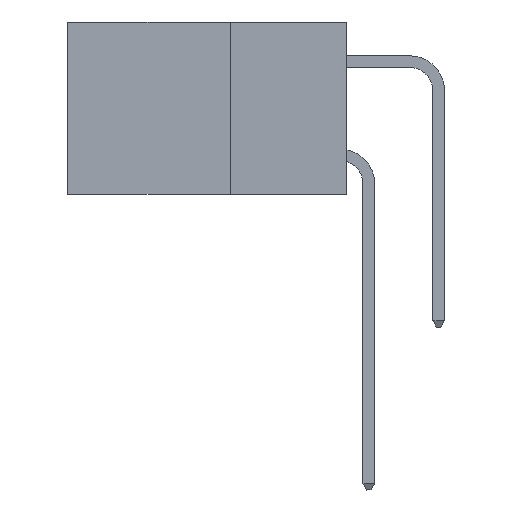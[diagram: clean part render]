
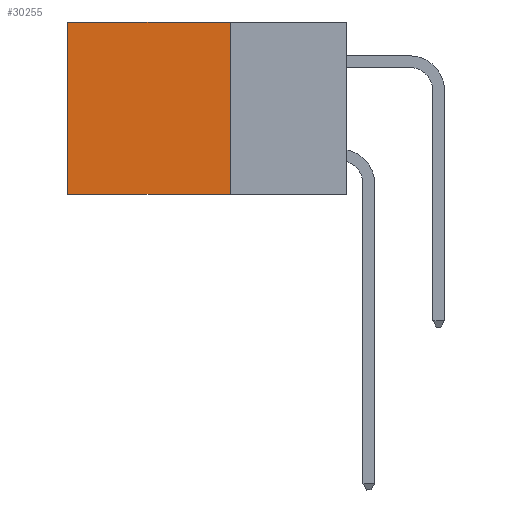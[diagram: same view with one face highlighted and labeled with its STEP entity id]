
A CAD part, left-side view. The second image highlights one B-rep face of the part: STEP entity #30255.
In plain terms, the highlighted planar face has unit normal (-1, 0, 0).
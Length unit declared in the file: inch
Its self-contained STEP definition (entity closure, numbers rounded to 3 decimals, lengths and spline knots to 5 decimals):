
#348 = VERTEX_POINT ( 'NONE', #10802 ) ;
#1206 = CARTESIAN_POINT ( 'NONE',  ( 0.2875, 0.25, 0. ) ) ;
#1921 = VECTOR ( 'NONE', #30288, 39.37008 ) ;
#4681 = EDGE_CURVE ( 'NONE', #19000, #29378, #31985, .T. ) ;
#5032 = DIRECTION ( 'NONE',  ( 1., 0., 0. ) ) ;
#6485 = EDGE_CURVE ( 'NONE', #29378, #12026, #27161, .T. ) ;
#6731 = VECTOR ( 'NONE', #34217, 39.37008 ) ;
#9121 = LINE ( 'NONE', #19174, #1921 ) ;
#9822 = ORIENTED_EDGE ( 'NONE', *, *, #4681, .F. ) ;
#9982 = CARTESIAN_POINT ( 'NONE',  ( 0.2875, 0.25, -0.37 ) ) ;
#10748 = FACE_OUTER_BOUND ( 'NONE', #27611, .T. ) ;
#10802 = CARTESIAN_POINT ( 'NONE',  ( 0.2875, 0.6, 0. ) ) ;
#10905 = EDGE_CURVE ( 'NONE', #348, #12026, #35286, .T. ) ;
#12026 = VERTEX_POINT ( 'NONE', #22882 ) ;
#12740 = EDGE_CURVE ( 'NONE', #19000, #348, #9121, .T. ) ;
#13282 = VECTOR ( 'NONE', #24494, 39.37008 ) ;
#14138 = ORIENTED_EDGE ( 'NONE', *, *, #10905, .T. ) ;
#14485 = DIRECTION ( 'NONE',  ( 0., 0., -1. ) ) ;
#15647 = VECTOR ( 'NONE', #14485, 39.37008 ) ;
#17063 = CARTESIAN_POINT ( 'NONE',  ( 0.2875, 0.25, -0.37 ) ) ;
#17558 = CARTESIAN_POINT ( 'NONE',  ( 0.2875, 0.25, 0. ) ) ;
#19000 = VERTEX_POINT ( 'NONE', #1206 ) ;
#19174 = CARTESIAN_POINT ( 'NONE',  ( 0.2875, 0.25, 0. ) ) ;
#20976 = DIRECTION ( 'NONE',  ( 0., 0., -1. ) ) ;
#22882 = CARTESIAN_POINT ( 'NONE',  ( 0.2875, 0.6, -0.37 ) ) ;
#23596 = PLANE ( 'NONE',  #23785 ) ;
#23785 = AXIS2_PLACEMENT_3D ( 'NONE', #34789, #5032, #20976 ) ;
#24494 = DIRECTION ( 'NONE',  ( 0., 0., -1. ) ) ;
#25568 = ORIENTED_EDGE ( 'NONE', *, *, #6485, .F. ) ;
#27161 = LINE ( 'NONE', #9982, #6731 ) ;
#27611 = EDGE_LOOP ( 'NONE', ( #14138, #25568, #9822, #29611 ) ) ;
#27710 = CARTESIAN_POINT ( 'NONE',  ( 0.2875, 0.6, 0. ) ) ;
#29378 = VERTEX_POINT ( 'NONE', #17063 ) ;
#29611 = ORIENTED_EDGE ( 'NONE', *, *, #12740, .T. ) ;
#30255 = ADVANCED_FACE ( 'NONE', ( #10748 ), #23596, .F. ) ;
#30288 = DIRECTION ( 'NONE',  ( 0., 1., 0. ) ) ;
#31985 = LINE ( 'NONE', #17558, #13282 ) ;
#34217 = DIRECTION ( 'NONE',  ( 0., 1., 0. ) ) ;
#34789 = CARTESIAN_POINT ( 'NONE',  ( 0.2875, 0.25, 0. ) ) ;
#35286 = LINE ( 'NONE', #27710, #15647 ) ;
